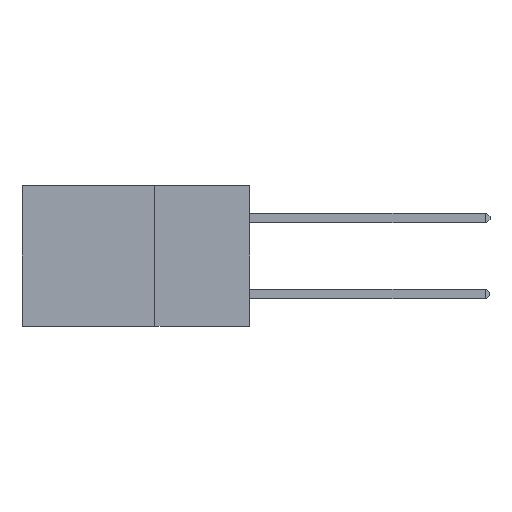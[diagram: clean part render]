
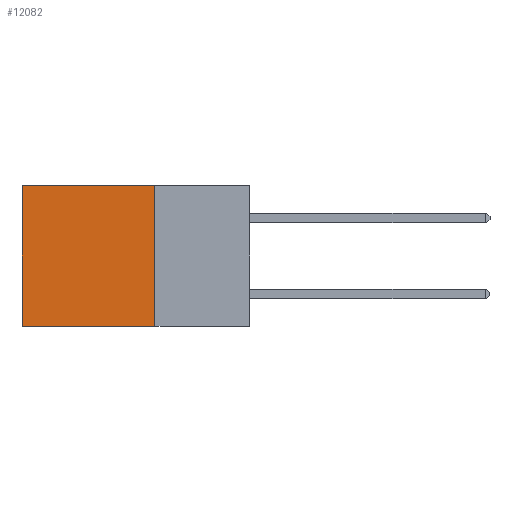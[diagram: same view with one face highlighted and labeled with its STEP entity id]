
A CAD part, left-side view. The second image highlights one B-rep face of the part: STEP entity #12082.
In plain terms, the highlighted planar face has unit normal (-1, 0, 0).
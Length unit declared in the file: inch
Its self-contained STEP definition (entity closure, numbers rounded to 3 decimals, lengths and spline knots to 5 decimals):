
#199 = ORIENTED_EDGE ( 'NONE', *, *, #19271, .F. ) ;
#325 = LINE ( 'NONE', #10657, #8767 ) ;
#1021 = DIRECTION ( 'NONE',  ( 1., 0., 0. ) ) ;
#2101 = EDGE_CURVE ( 'NONE', #11741, #19738, #10608, .T. ) ;
#2820 = CARTESIAN_POINT ( 'NONE',  ( 0.2875, 0.25, -0.37 ) ) ;
#3184 = VERTEX_POINT ( 'NONE', #5248 ) ;
#3671 = CARTESIAN_POINT ( 'NONE',  ( 0.2875, 0.6, 0. ) ) ;
#4025 = ORIENTED_EDGE ( 'NONE', *, *, #17902, .T. ) ;
#5248 = CARTESIAN_POINT ( 'NONE',  ( 0.2875, 0.6, -0.37 ) ) ;
#6463 = VECTOR ( 'NONE', #16415, 39.37008 ) ;
#6674 = CARTESIAN_POINT ( 'NONE',  ( 0.2875, 0.25, -0.37 ) ) ;
#6901 = FACE_OUTER_BOUND ( 'NONE', #14353, .T. ) ;
#7580 = VECTOR ( 'NONE', #9871, 39.37008 ) ;
#7751 = CARTESIAN_POINT ( 'NONE',  ( 0.2875, 0.25, 0. ) ) ;
#8499 = CARTESIAN_POINT ( 'NONE',  ( 0.2875, 0.25, 0. ) ) ;
#8767 = VECTOR ( 'NONE', #12286, 39.37008 ) ;
#9400 = PLANE ( 'NONE',  #9901 ) ;
#9871 = DIRECTION ( 'NONE',  ( 0., 1., 0. ) ) ;
#9901 = AXIS2_PLACEMENT_3D ( 'NONE', #20710, #1021, #12647 ) ;
#10608 = LINE ( 'NONE', #7751, #19695 ) ;
#10657 = CARTESIAN_POINT ( 'NONE',  ( 0.2875, 0.6, 0. ) ) ;
#10833 = LINE ( 'NONE', #6674, #6463 ) ;
#10953 = DIRECTION ( 'NONE',  ( 0., 0., -1. ) ) ;
#11741 = VERTEX_POINT ( 'NONE', #8499 ) ;
#12082 = ADVANCED_FACE ( 'NONE', ( #6901 ), #9400, .F. ) ;
#12286 = DIRECTION ( 'NONE',  ( 0., 0., -1. ) ) ;
#12647 = DIRECTION ( 'NONE',  ( 0., 0., -1. ) ) ;
#14152 = ORIENTED_EDGE ( 'NONE', *, *, #20245, .T. ) ;
#14353 = EDGE_LOOP ( 'NONE', ( #14152, #199, #14412, #4025 ) ) ;
#14412 = ORIENTED_EDGE ( 'NONE', *, *, #2101, .F. ) ;
#16415 = DIRECTION ( 'NONE',  ( 0., 1., 0. ) ) ;
#17424 = VERTEX_POINT ( 'NONE', #3671 ) ;
#17902 = EDGE_CURVE ( 'NONE', #11741, #17424, #19981, .T. ) ;
#19271 = EDGE_CURVE ( 'NONE', #19738, #3184, #10833, .T. ) ;
#19543 = CARTESIAN_POINT ( 'NONE',  ( 0.2875, 0.25, 0. ) ) ;
#19695 = VECTOR ( 'NONE', #10953, 39.37008 ) ;
#19738 = VERTEX_POINT ( 'NONE', #2820 ) ;
#19981 = LINE ( 'NONE', #19543, #7580 ) ;
#20245 = EDGE_CURVE ( 'NONE', #17424, #3184, #325, .T. ) ;
#20710 = CARTESIAN_POINT ( 'NONE',  ( 0.2875, 0.25, 0. ) ) ;
